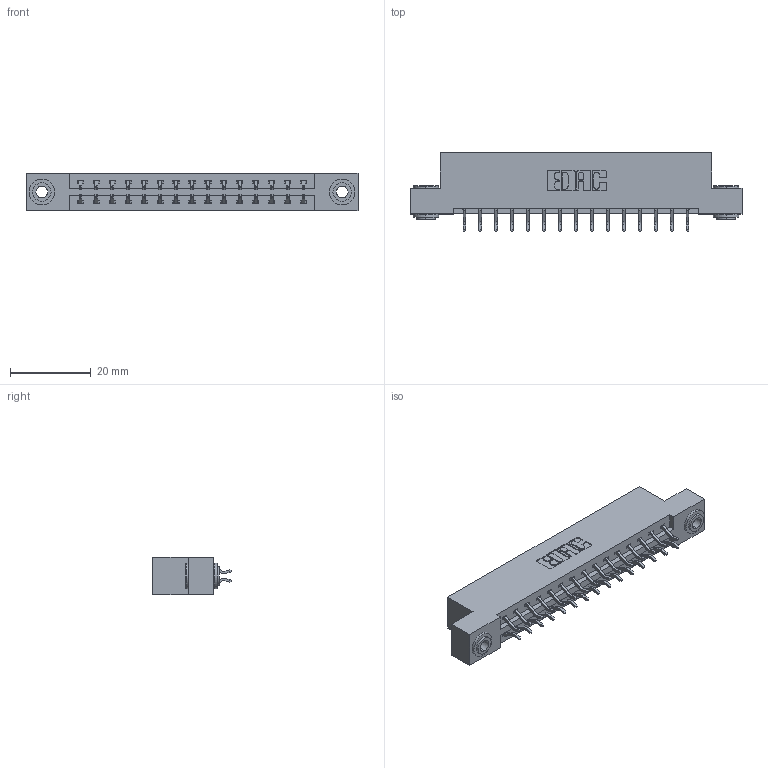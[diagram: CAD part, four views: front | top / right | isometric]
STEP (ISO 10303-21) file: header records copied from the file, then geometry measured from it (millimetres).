
FILE_DESCRIPTION (( 'STEP AP203' ), '1' );
FILE_NAME ('387-030-556-203.STEP', '2019-10-17T14:54:39', ( '' ), ( '' ), 'SwSTEP 2.0', 'SolidWorks 2016', '' );
FILE_SCHEMA (( 'CONFIG_CONTROL_DESIGN' ));
Length unit declared in the file: inch
Products named in the file (4): 337 Part_Flush Mounting Lugs - 0.156 Dia-TH; 345-292-001_556 Tail; 345-250-002_345-250-002-102; 387-030-556-203
Assembly tree (33 placements, depth 2):
  387-030-556-203
    337 Part_Flush Mounting Lugs - 0.156 Dia-TH
    345-292-001_556 Tail  x30
    345-250-002_345-250-002-102  x2
Bounding box: 82.45 x 19.57 x 9.4 mm (x, y, z)
Volume: 8347.9 mm3; surface area: 9367.8 mm2
Topology: 33 solids, 33 shells, 1952 faces, 5757 edges, 3794 vertices
Faces by surface type: plane 1340, cylinder 604, cone 8
Entity records: 15992 total; most frequent: CARTESIAN_POINT 2705, ORIENTED_EDGE 2622, DIRECTION 2373, EDGE_CURVE 1311, LINE 1151, VECTOR 1151, VERTEX_POINT 870, AXIS2_PLACEMENT_3D 611
